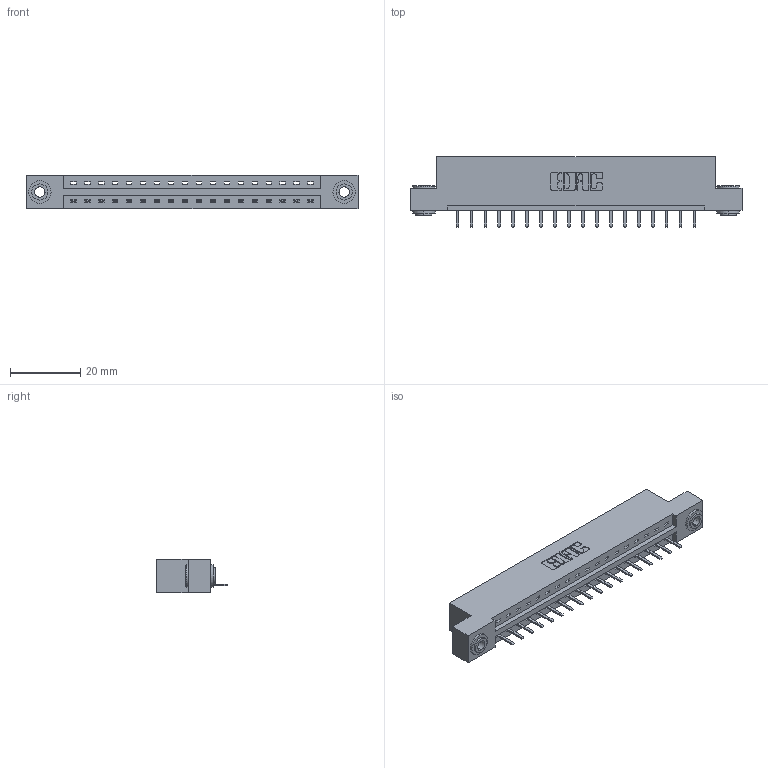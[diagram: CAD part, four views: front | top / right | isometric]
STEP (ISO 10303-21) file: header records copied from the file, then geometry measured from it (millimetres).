
FILE_DESCRIPTION (( 'STEP AP203' ), '1' );
FILE_NAME ('387-018-520-103.STEP', '2019-10-02T19:47:06', ( '' ), ( '' ), 'SwSTEP 2.0', 'SolidWorks 2016', '' );
FILE_SCHEMA (( 'CONFIG_CONTROL_DESIGN' ));
Length unit declared in the file: inch
Products named in the file (4): 387-018-520-103; 345-250-002_345-250-002-102; 337 Part_Flush Mounting Lugs - 0.156 Dia-TH; 345-292-001_345-293-120
Assembly tree (21 placements, depth 2):
  387-018-520-103
    337 Part_Flush Mounting Lugs - 0.156 Dia-TH
    345-292-001_345-293-120  x18
    345-250-002_345-250-002-102  x2
Bounding box: 94.34 x 20.02 x 9.4 mm (x, y, z)
Volume: 9471.9 mm3; surface area: 9700.9 mm2
Topology: 21 solids, 21 shells, 1340 faces, 3915 edges, 2558 vertices
Faces by surface type: plane 944, cylinder 388, cone 8
Entity records: 17248 total; most frequent: CARTESIAN_POINT 2991, ORIENTED_EDGE 2926, DIRECTION 2589, EDGE_CURVE 1463, VECTOR 1307, LINE 1307, VERTEX_POINT 970, AXIS2_PLACEMENT_3D 641
